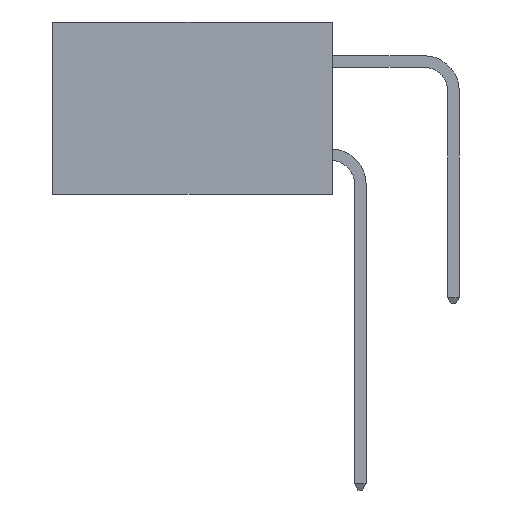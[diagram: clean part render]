
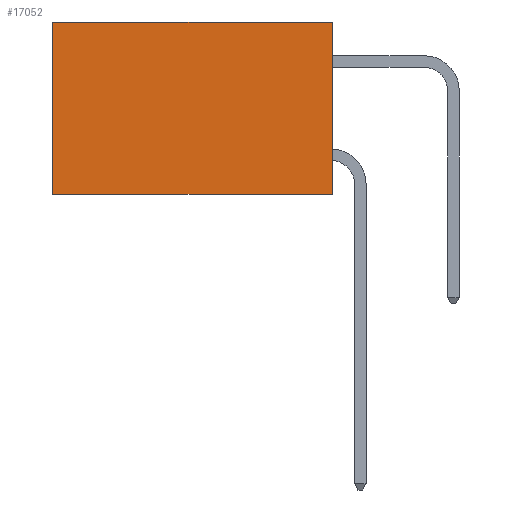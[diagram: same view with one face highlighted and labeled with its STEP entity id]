
A CAD part, left-side view. The second image highlights one B-rep face of the part: STEP entity #17052.
In plain terms, the highlighted planar face has unit normal (-1, 0, 0).
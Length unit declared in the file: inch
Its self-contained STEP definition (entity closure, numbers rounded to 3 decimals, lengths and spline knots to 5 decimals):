
#446 = LINE ( 'NONE', #7651, #5066 ) ;
#1077 = LINE ( 'NONE', #3716, #14329 ) ;
#1208 = DIRECTION ( 'NONE',  ( 0., 1., 0. ) ) ;
#1778 = LINE ( 'NONE', #6353, #19165 ) ;
#1789 = EDGE_CURVE ( 'NONE', #18596, #13277, #16330, .T. ) ;
#1985 = VERTEX_POINT ( 'NONE', #21701 ) ;
#2035 = CARTESIAN_POINT ( 'NONE',  ( 0.298, 0.6, -0.37 ) ) ;
#2043 = DIRECTION ( 'NONE',  ( 0., 0., -1. ) ) ;
#2479 = DIRECTION ( 'NONE',  ( 0., 1., 0. ) ) ;
#2509 = VECTOR ( 'NONE', #5622, 39.37008 ) ;
#2870 = PLANE ( 'NONE',  #15652 ) ;
#3716 = CARTESIAN_POINT ( 'NONE',  ( 0.298, 0., 0. ) ) ;
#5066 = VECTOR ( 'NONE', #2479, 39.37008 ) ;
#5622 = DIRECTION ( 'NONE',  ( 0., 0., -1. ) ) ;
#6305 = CARTESIAN_POINT ( 'NONE',  ( 0.298, 0., 0. ) ) ;
#6353 = CARTESIAN_POINT ( 'NONE',  ( 0.298, 0., -0.37 ) ) ;
#6376 = DIRECTION ( 'NONE',  ( 0., 0., -1. ) ) ;
#7168 = VERTEX_POINT ( 'NONE', #19919 ) ;
#7651 = CARTESIAN_POINT ( 'NONE',  ( 0.298, 0., 0. ) ) ;
#8184 = EDGE_CURVE ( 'NONE', #1985, #7168, #1077, .T. ) ;
#9100 = ORIENTED_EDGE ( 'NONE', *, *, #1789, .T. ) ;
#9231 = FACE_OUTER_BOUND ( 'NONE', #19808, .T. ) ;
#12139 = ORIENTED_EDGE ( 'NONE', *, *, #19167, .T. ) ;
#12371 = ORIENTED_EDGE ( 'NONE', *, *, #19349, .F. ) ;
#13277 = VERTEX_POINT ( 'NONE', #2035 ) ;
#14329 = VECTOR ( 'NONE', #2043, 39.37008 ) ;
#14331 = CARTESIAN_POINT ( 'NONE',  ( 0.298, 0.6, 0. ) ) ;
#15652 = AXIS2_PLACEMENT_3D ( 'NONE', #6305, #16755, #6376 ) ;
#15971 = ORIENTED_EDGE ( 'NONE', *, *, #8184, .F. ) ;
#16330 = LINE ( 'NONE', #14331, #2509 ) ;
#16755 = DIRECTION ( 'NONE',  ( 1., 0., 0. ) ) ;
#17052 = ADVANCED_FACE ( 'NONE', ( #9231 ), #2870, .F. ) ;
#18596 = VERTEX_POINT ( 'NONE', #20064 ) ;
#19165 = VECTOR ( 'NONE', #1208, 39.37008 ) ;
#19167 = EDGE_CURVE ( 'NONE', #1985, #18596, #446, .T. ) ;
#19349 = EDGE_CURVE ( 'NONE', #7168, #13277, #1778, .T. ) ;
#19808 = EDGE_LOOP ( 'NONE', ( #9100, #12371, #15971, #12139 ) ) ;
#19919 = CARTESIAN_POINT ( 'NONE',  ( 0.298, 0., -0.37 ) ) ;
#20064 = CARTESIAN_POINT ( 'NONE',  ( 0.298, 0.6, 0. ) ) ;
#21701 = CARTESIAN_POINT ( 'NONE',  ( 0.298, 0., 0. ) ) ;
